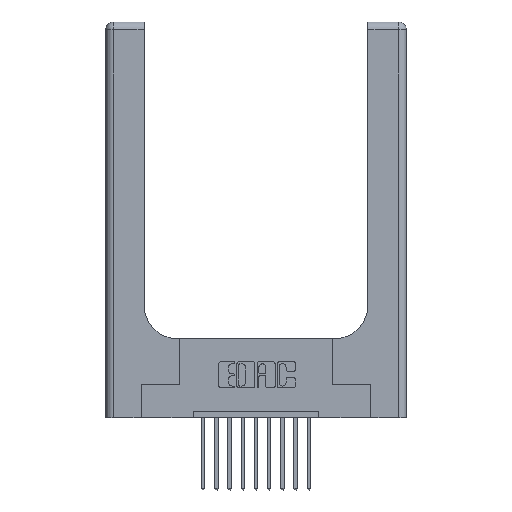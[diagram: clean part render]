
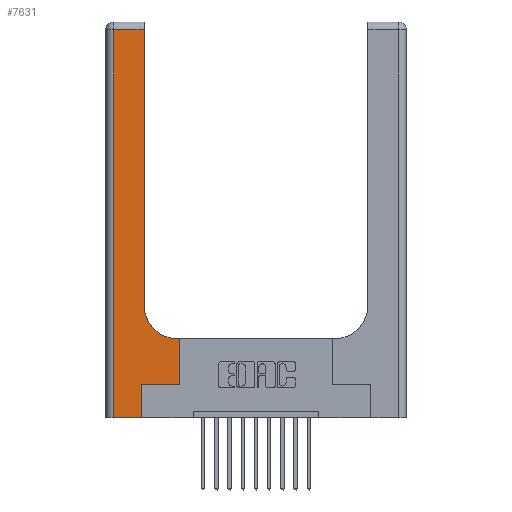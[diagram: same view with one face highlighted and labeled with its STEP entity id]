
A CAD part, top view. The second image highlights one B-rep face of the part: STEP entity #7631.
In plain terms, the highlighted planar face has unit normal (0, 0, 1).
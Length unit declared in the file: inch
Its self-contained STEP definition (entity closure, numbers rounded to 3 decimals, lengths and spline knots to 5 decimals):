
#548 = VERTEX_POINT ( 'NONE', #15860 ) ;
#664 = DIRECTION ( 'NONE',  ( 0., 0., -1. ) ) ;
#728 = LINE ( 'NONE', #5075, #4255 ) ;
#982 = VERTEX_POINT ( 'NONE', #13142 ) ;
#1291 = ORIENTED_EDGE ( 'NONE', *, *, #10873, .T. ) ;
#1371 = EDGE_LOOP ( 'NONE', ( #2950, #10088, #6545, #8378, #2839, #13455, #1291, #7274, #8437 ) ) ;
#1789 = DIRECTION ( 'NONE',  ( 1., 0., 0. ) ) ;
#1835 = DIRECTION ( 'NONE',  ( 0., -1., 0. ) ) ;
#1942 = DIRECTION ( 'NONE',  ( -1., 0., 0. ) ) ;
#2710 = CARTESIAN_POINT ( 'NONE',  ( 0.269, 0., 0.37 ) ) ;
#2839 = ORIENTED_EDGE ( 'NONE', *, *, #7128, .T. ) ;
#2950 = ORIENTED_EDGE ( 'NONE', *, *, #4527, .T. ) ;
#3075 = VERTEX_POINT ( 'NONE', #7252 ) ;
#3101 = PLANE ( 'NONE',  #3838 ) ;
#3437 = CARTESIAN_POINT ( 'NONE',  ( 0.5415, 0.85, 0.37 ) ) ;
#3838 = AXIS2_PLACEMENT_3D ( 'NONE', #10581, #664, #1942 ) ;
#4254 = EDGE_CURVE ( 'NONE', #982, #4823, #10656, .T. ) ;
#4255 = VECTOR ( 'NONE', #6239, 39.37008 ) ;
#4457 = CARTESIAN_POINT ( 'NONE',  ( 0.06, 3., 0.37 ) ) ;
#4527 = EDGE_CURVE ( 'NONE', #3075, #7798, #5495, .T. ) ;
#4672 = DIRECTION ( 'NONE',  ( 0., 0., -1. ) ) ;
#4823 = VERTEX_POINT ( 'NONE', #10357 ) ;
#5075 = CARTESIAN_POINT ( 'NONE',  ( 0.269, 0., 0.37 ) ) ;
#5324 = AXIS2_PLACEMENT_3D ( 'NONE', #3437, #4672, #5951 ) ;
#5443 = CARTESIAN_POINT ( 'NONE',  ( 0.2915, 0.6, 0.37 ) ) ;
#5495 = LINE ( 'NONE', #8915, #11863 ) ;
#5864 = LINE ( 'NONE', #4457, #8413 ) ;
#5951 = DIRECTION ( 'NONE',  ( 1., 0., 0. ) ) ;
#6131 = EDGE_CURVE ( 'NONE', #7798, #12349, #9407, .T. ) ;
#6239 = DIRECTION ( 'NONE',  ( 0., 1., 0. ) ) ;
#6545 = ORIENTED_EDGE ( 'NONE', *, *, #12538, .T. ) ;
#7128 = EDGE_CURVE ( 'NONE', #9860, #982, #728, .T. ) ;
#7252 = CARTESIAN_POINT ( 'NONE',  ( 0.2915, 0.85, 0.37 ) ) ;
#7274 = ORIENTED_EDGE ( 'NONE', *, *, #8983, .T. ) ;
#7631 = ADVANCED_FACE ( 'NONE', ( #15779 ), #3101, .F. ) ;
#7758 = CARTESIAN_POINT ( 'NONE',  ( 0.06, 2.94, 0.37 ) ) ;
#7798 = VERTEX_POINT ( 'NONE', #15114 ) ;
#8008 = VERTEX_POINT ( 'NONE', #15436 ) ;
#8277 = VECTOR ( 'NONE', #13415, 39.37008 ) ;
#8283 = LINE ( 'NONE', #10386, #15060 ) ;
#8378 = ORIENTED_EDGE ( 'NONE', *, *, #9332, .T. ) ;
#8413 = VECTOR ( 'NONE', #1835, 39.37008 ) ;
#8437 = ORIENTED_EDGE ( 'NONE', *, *, #10630, .T. ) ;
#8915 = CARTESIAN_POINT ( 'NONE',  ( 0.2915, 3., 0.37 ) ) ;
#8983 = EDGE_CURVE ( 'NONE', #15249, #548, #14922, .T. ) ;
#9112 = DIRECTION ( 'NONE',  ( 0., 1., 0. ) ) ;
#9213 = CARTESIAN_POINT ( 'NONE',  ( 0., 0., 0.37 ) ) ;
#9332 = EDGE_CURVE ( 'NONE', #8008, #9860, #15920, .T. ) ;
#9407 = LINE ( 'NONE', #12593, #13985 ) ;
#9860 = VERTEX_POINT ( 'NONE', #2710 ) ;
#9979 = DIRECTION ( 'NONE',  ( 0., 1., 0. ) ) ;
#10088 = ORIENTED_EDGE ( 'NONE', *, *, #6131, .T. ) ;
#10131 = DIRECTION ( 'NONE',  ( -1., 0., 0. ) ) ;
#10357 = CARTESIAN_POINT ( 'NONE',  ( 0.5585, 0.25, 0.37 ) ) ;
#10386 = CARTESIAN_POINT ( 'NONE',  ( 0.5585, 0.25, 0.37 ) ) ;
#10581 = CARTESIAN_POINT ( 'NONE',  ( 0., 3., 0.37 ) ) ;
#10630 = EDGE_CURVE ( 'NONE', #548, #3075, #11882, .T. ) ;
#10656 = LINE ( 'NONE', #12143, #8277 ) ;
#10873 = EDGE_CURVE ( 'NONE', #4823, #15249, #8283, .T. ) ;
#10924 = VECTOR ( 'NONE', #11735, 39.37008 ) ;
#11454 = CARTESIAN_POINT ( 'NONE',  ( 0.5585, 0.6, 0.37 ) ) ;
#11735 = DIRECTION ( 'NONE',  ( -1., 0., 0. ) ) ;
#11863 = VECTOR ( 'NONE', #9979, 39.37008 ) ;
#11882 = CIRCLE ( 'NONE', #5324, 0.25 ) ;
#12143 = CARTESIAN_POINT ( 'NONE',  ( 0.269, 0.25, 0.37 ) ) ;
#12349 = VERTEX_POINT ( 'NONE', #7758 ) ;
#12526 = VECTOR ( 'NONE', #1789, 39.37008 ) ;
#12538 = EDGE_CURVE ( 'NONE', #12349, #8008, #5864, .T. ) ;
#12593 = CARTESIAN_POINT ( 'NONE',  ( 0., 2.94, 0.37 ) ) ;
#13142 = CARTESIAN_POINT ( 'NONE',  ( 0.269, 0.25, 0.37 ) ) ;
#13415 = DIRECTION ( 'NONE',  ( 1., 0., 0. ) ) ;
#13455 = ORIENTED_EDGE ( 'NONE', *, *, #4254, .T. ) ;
#13985 = VECTOR ( 'NONE', #10131, 39.37008 ) ;
#14922 = LINE ( 'NONE', #5443, #10924 ) ;
#15060 = VECTOR ( 'NONE', #9112, 39.37008 ) ;
#15114 = CARTESIAN_POINT ( 'NONE',  ( 0.2915, 2.94, 0.37 ) ) ;
#15249 = VERTEX_POINT ( 'NONE', #11454 ) ;
#15436 = CARTESIAN_POINT ( 'NONE',  ( 0.06, 0., 0.37 ) ) ;
#15779 = FACE_OUTER_BOUND ( 'NONE', #1371, .T. ) ;
#15860 = CARTESIAN_POINT ( 'NONE',  ( 0.5415, 0.6, 0.37 ) ) ;
#15920 = LINE ( 'NONE', #9213, #12526 ) ;
